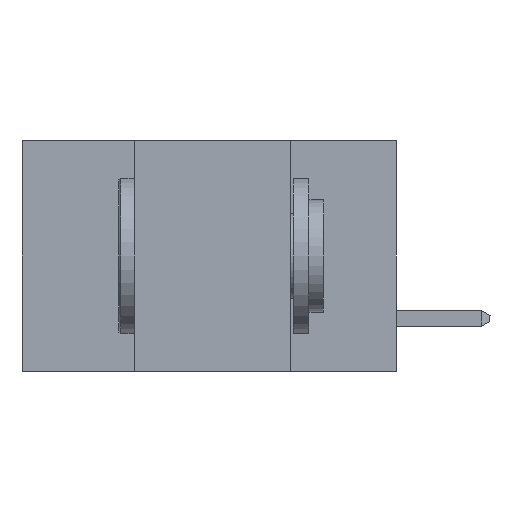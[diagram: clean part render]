
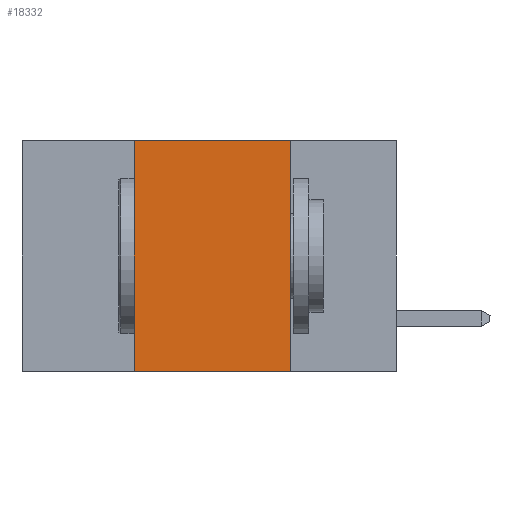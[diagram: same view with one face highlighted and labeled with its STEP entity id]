
A CAD part, left-side view. The second image highlights one B-rep face of the part: STEP entity #18332.
In plain terms, the highlighted planar face has unit normal (-1, 0, 0).
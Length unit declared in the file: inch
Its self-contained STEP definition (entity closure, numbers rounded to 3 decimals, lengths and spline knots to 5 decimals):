
#958 = ORIENTED_EDGE ( 'NONE', *, *, #6888, .F. ) ;
#2457 = VERTEX_POINT ( 'NONE', #18647 ) ;
#3023 = PLANE ( 'NONE',  #24954 ) ;
#5003 = DIRECTION ( 'NONE',  ( 0., -1., 0. ) ) ;
#5052 = CARTESIAN_POINT ( 'NONE',  ( 0., 0.6, 0. ) ) ;
#5210 = VECTOR ( 'NONE', #25701, 39.37008 ) ;
#5536 = EDGE_CURVE ( 'NONE', #2457, #9070, #19120, .T. ) ;
#5844 = CARTESIAN_POINT ( 'NONE',  ( 0., 0.6, -0.37 ) ) ;
#6031 = ORIENTED_EDGE ( 'NONE', *, *, #14627, .F. ) ;
#6039 = LINE ( 'NONE', #23162, #6599 ) ;
#6599 = VECTOR ( 'NONE', #13191, 39.37008 ) ;
#6631 = VECTOR ( 'NONE', #16948, 39.37008 ) ;
#6888 = EDGE_CURVE ( 'NONE', #2457, #7260, #13359, .T. ) ;
#7002 = VERTEX_POINT ( 'NONE', #16630 ) ;
#7084 = DIRECTION ( 'NONE',  ( 1., 0., 0. ) ) ;
#7260 = VERTEX_POINT ( 'NONE', #15027 ) ;
#7662 = ORIENTED_EDGE ( 'NONE', *, *, #5536, .T. ) ;
#7745 = CARTESIAN_POINT ( 'NONE',  ( 0., 0.17, -0.37 ) ) ;
#9070 = VERTEX_POINT ( 'NONE', #25558 ) ;
#13191 = DIRECTION ( 'NONE',  ( 0., -1., 0. ) ) ;
#13272 = EDGE_CURVE ( 'NONE', #7260, #7002, #6039, .T. ) ;
#13359 = LINE ( 'NONE', #16980, #6631 ) ;
#13766 = VECTOR ( 'NONE', #5003, 39.37008 ) ;
#14627 = EDGE_CURVE ( 'NONE', #7002, #9070, #16031, .T. ) ;
#15027 = CARTESIAN_POINT ( 'NONE',  ( 0., 0.42, 0. ) ) ;
#16031 = LINE ( 'NONE', #7745, #5210 ) ;
#16630 = CARTESIAN_POINT ( 'NONE',  ( 0., 0.17, 0. ) ) ;
#16948 = DIRECTION ( 'NONE',  ( 0., 0., 1. ) ) ;
#16980 = CARTESIAN_POINT ( 'NONE',  ( 0., 0.42, -0.37 ) ) ;
#18111 = ORIENTED_EDGE ( 'NONE', *, *, #13272, .F. ) ;
#18332 = ADVANCED_FACE ( 'NONE', ( #25095 ), #3023, .F. ) ;
#18647 = CARTESIAN_POINT ( 'NONE',  ( 0., 0.42, -0.37 ) ) ;
#19120 = LINE ( 'NONE', #5844, #13766 ) ;
#21188 = DIRECTION ( 'NONE',  ( 0., 0., -1. ) ) ;
#23162 = CARTESIAN_POINT ( 'NONE',  ( 0., 0.6, 0. ) ) ;
#24954 = AXIS2_PLACEMENT_3D ( 'NONE', #5052, #7084, #21188 ) ;
#25095 = FACE_OUTER_BOUND ( 'NONE', #25524, .T. ) ;
#25524 = EDGE_LOOP ( 'NONE', ( #6031, #18111, #958, #7662 ) ) ;
#25558 = CARTESIAN_POINT ( 'NONE',  ( 0., 0.17, -0.37 ) ) ;
#25701 = DIRECTION ( 'NONE',  ( 0., 0., -1. ) ) ;
